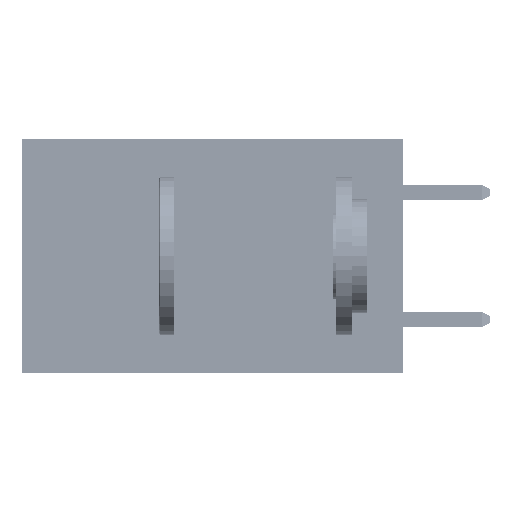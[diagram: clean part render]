
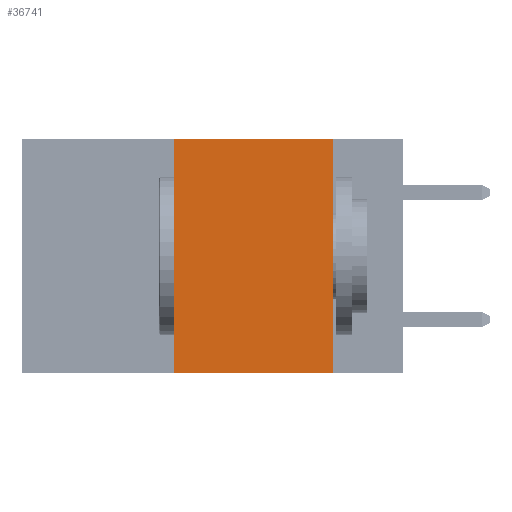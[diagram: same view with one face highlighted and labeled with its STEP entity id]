
A CAD part, left-side view. The second image highlights one B-rep face of the part: STEP entity #36741.
In plain terms, the highlighted planar face has unit normal (-1, 0, 0).
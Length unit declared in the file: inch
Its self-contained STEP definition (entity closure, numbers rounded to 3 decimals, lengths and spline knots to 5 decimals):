
#3282 = CARTESIAN_POINT ( 'NONE',  ( 0., 0.6, 0. ) ) ;
#4507 = EDGE_CURVE ( 'NONE', #9803, #29019, #6105, .T. ) ;
#5358 = VECTOR ( 'NONE', #9412, 39.37008 ) ;
#6105 = LINE ( 'NONE', #8901, #29635 ) ;
#7504 = DIRECTION ( 'NONE',  ( 0., -1., 0. ) ) ;
#8167 = VERTEX_POINT ( 'NONE', #28495 ) ;
#8717 = DIRECTION ( 'NONE',  ( 0., 0., 1. ) ) ;
#8901 = CARTESIAN_POINT ( 'NONE',  ( 0., 0.36, 0. ) ) ;
#9412 = DIRECTION ( 'NONE',  ( 0., -1., 0. ) ) ;
#9664 = EDGE_CURVE ( 'NONE', #8167, #24432, #50401, .T. ) ;
#9689 = DIRECTION ( 'NONE',  ( 0., 0., -1. ) ) ;
#9803 = VERTEX_POINT ( 'NONE', #52599 ) ;
#11821 = CARTESIAN_POINT ( 'NONE',  ( 0., 0.11, -0.37 ) ) ;
#15421 = EDGE_CURVE ( 'NONE', #9803, #24432, #15529, .T. ) ;
#15529 = LINE ( 'NONE', #25425, #5358 ) ;
#21310 = CARTESIAN_POINT ( 'NONE',  ( 0., 0.11, 0. ) ) ;
#21978 = PLANE ( 'NONE',  #40027 ) ;
#24432 = VERTEX_POINT ( 'NONE', #11821 ) ;
#25358 = DIRECTION ( 'NONE',  ( 0., 0., -1. ) ) ;
#25425 = CARTESIAN_POINT ( 'NONE',  ( 0., 0.6, -0.37 ) ) ;
#28495 = CARTESIAN_POINT ( 'NONE',  ( 0., 0.11, 0. ) ) ;
#28656 = ORIENTED_EDGE ( 'NONE', *, *, #15421, .T. ) ;
#29019 = VERTEX_POINT ( 'NONE', #39549 ) ;
#29371 = VECTOR ( 'NONE', #25358, 39.37008 ) ;
#29635 = VECTOR ( 'NONE', #8717, 39.37008 ) ;
#30055 = ORIENTED_EDGE ( 'NONE', *, *, #47812, .F. ) ;
#34038 = CARTESIAN_POINT ( 'NONE',  ( 0., 0.6, 0. ) ) ;
#34981 = ORIENTED_EDGE ( 'NONE', *, *, #9664, .F. ) ;
#36643 = ORIENTED_EDGE ( 'NONE', *, *, #4507, .F. ) ;
#36741 = ADVANCED_FACE ( 'NONE', ( #43691 ), #21978, .F. ) ;
#37944 = DIRECTION ( 'NONE',  ( 1., 0., 0. ) ) ;
#39549 = CARTESIAN_POINT ( 'NONE',  ( 0., 0.36, 0. ) ) ;
#40027 = AXIS2_PLACEMENT_3D ( 'NONE', #34038, #37944, #9689 ) ;
#42814 = LINE ( 'NONE', #3282, #52385 ) ;
#43491 = EDGE_LOOP ( 'NONE', ( #34981, #30055, #36643, #28656 ) ) ;
#43691 = FACE_OUTER_BOUND ( 'NONE', #43491, .T. ) ;
#47812 = EDGE_CURVE ( 'NONE', #29019, #8167, #42814, .T. ) ;
#50401 = LINE ( 'NONE', #21310, #29371 ) ;
#52385 = VECTOR ( 'NONE', #7504, 39.37008 ) ;
#52599 = CARTESIAN_POINT ( 'NONE',  ( 0., 0.36, -0.37 ) ) ;
